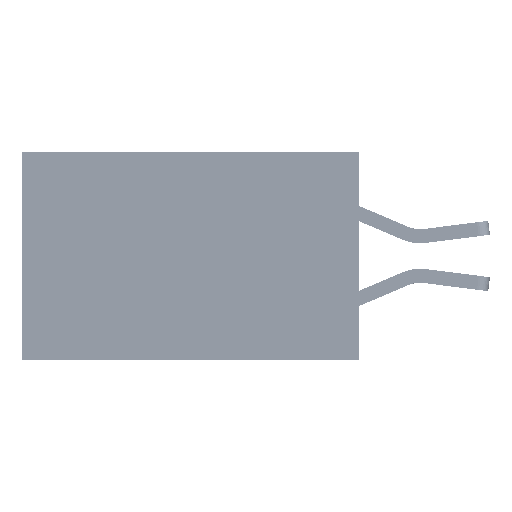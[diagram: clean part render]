
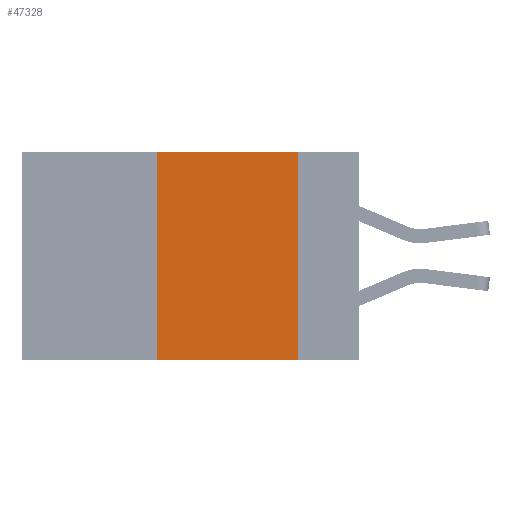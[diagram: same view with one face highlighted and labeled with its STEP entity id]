
A CAD part, left-side view. The second image highlights one B-rep face of the part: STEP entity #47328.
In plain terms, the highlighted planar face has unit normal (-1, 0, 0).
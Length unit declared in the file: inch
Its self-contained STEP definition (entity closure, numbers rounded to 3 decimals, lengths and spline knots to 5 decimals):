
#3668 = VERTEX_POINT ( 'NONE', #52938 ) ;
#3899 = CARTESIAN_POINT ( 'NONE',  ( 0., 0.11, 0. ) ) ;
#4880 = AXIS2_PLACEMENT_3D ( 'NONE', #38828, #6138, #14534 ) ;
#5227 = VECTOR ( 'NONE', #22141, 39.37008 ) ;
#6138 = DIRECTION ( 'NONE',  ( 1., 0., 0. ) ) ;
#6518 = EDGE_CURVE ( 'NONE', #31639, #3668, #29264, .T. ) ;
#12338 = ORIENTED_EDGE ( 'NONE', *, *, #40153, .F. ) ;
#14534 = DIRECTION ( 'NONE',  ( 0., 0., -1. ) ) ;
#16586 = CARTESIAN_POINT ( 'NONE',  ( 0., 0.6, -0.37 ) ) ;
#18101 = EDGE_LOOP ( 'NONE', ( #12338, #31258, #42780, #52066 ) ) ;
#18891 = LINE ( 'NONE', #51810, #46448 ) ;
#19110 = CARTESIAN_POINT ( 'NONE',  ( 0., 0.36, -0.37 ) ) ;
#22141 = DIRECTION ( 'NONE',  ( 0., 0., -1. ) ) ;
#23789 = DIRECTION ( 'NONE',  ( 0., -1., 0. ) ) ;
#26709 = FACE_OUTER_BOUND ( 'NONE', #18101, .T. ) ;
#27707 = VERTEX_POINT ( 'NONE', #3899 ) ;
#28173 = VECTOR ( 'NONE', #41943, 39.37008 ) ;
#29264 = LINE ( 'NONE', #16586, #28173 ) ;
#29697 = LINE ( 'NONE', #49964, #5227 ) ;
#30476 = PLANE ( 'NONE',  #4880 ) ;
#31258 = ORIENTED_EDGE ( 'NONE', *, *, #35028, .F. ) ;
#31279 = DIRECTION ( 'NONE',  ( 0., 0., 1. ) ) ;
#31639 = VERTEX_POINT ( 'NONE', #19110 ) ;
#33772 = VERTEX_POINT ( 'NONE', #40459 ) ;
#35028 = EDGE_CURVE ( 'NONE', #33772, #27707, #36192, .T. ) ;
#35372 = EDGE_CURVE ( 'NONE', #31639, #33772, #18891, .T. ) ;
#36192 = LINE ( 'NONE', #37003, #47248 ) ;
#37003 = CARTESIAN_POINT ( 'NONE',  ( 0., 0.6, 0. ) ) ;
#38828 = CARTESIAN_POINT ( 'NONE',  ( 0., 0.6, 0. ) ) ;
#40153 = EDGE_CURVE ( 'NONE', #27707, #3668, #29697, .T. ) ;
#40459 = CARTESIAN_POINT ( 'NONE',  ( 0., 0.36, 0. ) ) ;
#41943 = DIRECTION ( 'NONE',  ( 0., -1., 0. ) ) ;
#42780 = ORIENTED_EDGE ( 'NONE', *, *, #35372, .F. ) ;
#46448 = VECTOR ( 'NONE', #31279, 39.37008 ) ;
#47248 = VECTOR ( 'NONE', #23789, 39.37008 ) ;
#47328 = ADVANCED_FACE ( 'NONE', ( #26709 ), #30476, .F. ) ;
#49964 = CARTESIAN_POINT ( 'NONE',  ( 0., 0.11, 0. ) ) ;
#51810 = CARTESIAN_POINT ( 'NONE',  ( 0., 0.36, 0. ) ) ;
#52066 = ORIENTED_EDGE ( 'NONE', *, *, #6518, .T. ) ;
#52938 = CARTESIAN_POINT ( 'NONE',  ( 0., 0.11, -0.37 ) ) ;
